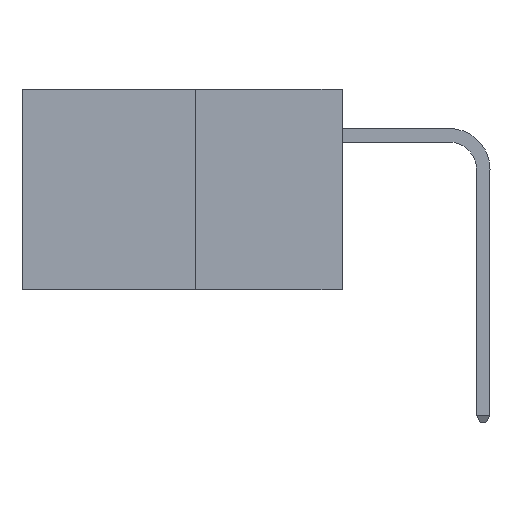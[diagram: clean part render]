
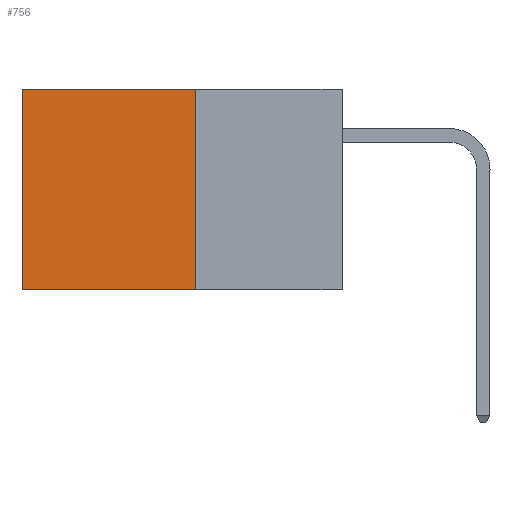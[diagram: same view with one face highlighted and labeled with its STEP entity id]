
A CAD part, left-side view. The second image highlights one B-rep face of the part: STEP entity #756.
In plain terms, the highlighted planar face has unit normal (-1, 0, 0).
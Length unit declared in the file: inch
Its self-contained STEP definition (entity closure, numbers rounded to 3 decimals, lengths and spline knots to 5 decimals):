
#80 = ORIENTED_EDGE ( 'NONE', *, *, #10915, .F. ) ;
#391 = DIRECTION ( 'NONE',  ( 0., 1., 0. ) ) ;
#556 = CARTESIAN_POINT ( 'NONE',  ( 0.277, 0.59, 0. ) ) ;
#756 = ADVANCED_FACE ( 'NONE', ( #16595 ), #7903, .F. ) ;
#1355 = VECTOR ( 'NONE', #12847, 39.37008 ) ;
#1972 = VECTOR ( 'NONE', #9024, 39.37008 ) ;
#2241 = VERTEX_POINT ( 'NONE', #6209 ) ;
#2269 = ORIENTED_EDGE ( 'NONE', *, *, #2438, .T. ) ;
#2438 = EDGE_CURVE ( 'NONE', #16931, #2241, #9279, .T. ) ;
#3084 = CARTESIAN_POINT ( 'NONE',  ( 0.277, 0.27, 0. ) ) ;
#3528 = DIRECTION ( 'NONE',  ( 0., 0., -1. ) ) ;
#4147 = CARTESIAN_POINT ( 'NONE',  ( 0.277, 0.27, -0.37 ) ) ;
#5098 = VERTEX_POINT ( 'NONE', #6888 ) ;
#5719 = LINE ( 'NONE', #16210, #16004 ) ;
#6209 = CARTESIAN_POINT ( 'NONE',  ( 0.277, 0.59, -0.37 ) ) ;
#6835 = EDGE_CURVE ( 'NONE', #5098, #2241, #5719, .T. ) ;
#6888 = CARTESIAN_POINT ( 'NONE',  ( 0.277, 0.27, -0.37 ) ) ;
#6966 = VECTOR ( 'NONE', #391, 39.37008 ) ;
#7091 = DIRECTION ( 'NONE',  ( 1., 0., 0. ) ) ;
#7903 = PLANE ( 'NONE',  #11591 ) ;
#7944 = ORIENTED_EDGE ( 'NONE', *, *, #16256, .T. ) ;
#9024 = DIRECTION ( 'NONE',  ( 0., 0., -1. ) ) ;
#9279 = LINE ( 'NONE', #11158, #1972 ) ;
#10714 = EDGE_LOOP ( 'NONE', ( #2269, #13157, #80, #7944 ) ) ;
#10915 = EDGE_CURVE ( 'NONE', #13144, #5098, #16147, .T. ) ;
#11158 = CARTESIAN_POINT ( 'NONE',  ( 0.277, 0.59, -0.37 ) ) ;
#11591 = AXIS2_PLACEMENT_3D ( 'NONE', #4147, #7091, #3528 ) ;
#12847 = DIRECTION ( 'NONE',  ( 0., 0., -1. ) ) ;
#13144 = VERTEX_POINT ( 'NONE', #3084 ) ;
#13157 = ORIENTED_EDGE ( 'NONE', *, *, #6835, .F. ) ;
#14037 = LINE ( 'NONE', #15269, #6966 ) ;
#14179 = CARTESIAN_POINT ( 'NONE',  ( 0.277, 0.27, -0.37 ) ) ;
#15269 = CARTESIAN_POINT ( 'NONE',  ( 0.277, 0.27, 0. ) ) ;
#15616 = DIRECTION ( 'NONE',  ( 0., 1., 0. ) ) ;
#16004 = VECTOR ( 'NONE', #15616, 39.37008 ) ;
#16147 = LINE ( 'NONE', #14179, #1355 ) ;
#16210 = CARTESIAN_POINT ( 'NONE',  ( 0.277, 0.27, -0.37 ) ) ;
#16256 = EDGE_CURVE ( 'NONE', #13144, #16931, #14037, .T. ) ;
#16595 = FACE_OUTER_BOUND ( 'NONE', #10714, .T. ) ;
#16931 = VERTEX_POINT ( 'NONE', #556 ) ;
